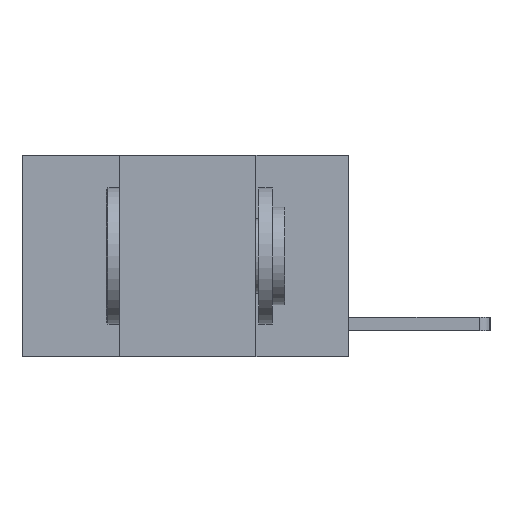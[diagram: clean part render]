
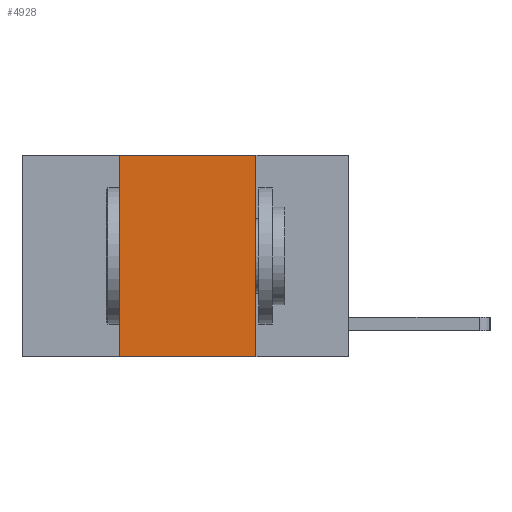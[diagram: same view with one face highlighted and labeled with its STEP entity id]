
A CAD part, left-side view. The second image highlights one B-rep face of the part: STEP entity #4928.
In plain terms, the highlighted planar face has unit normal (-1, 0, 0).
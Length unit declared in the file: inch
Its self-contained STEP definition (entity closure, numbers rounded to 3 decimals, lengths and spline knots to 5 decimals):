
#73 = LINE ( 'NONE', #692, #1565 ) ;
#147 = FACE_OUTER_BOUND ( 'NONE', #487, .T. ) ;
#232 = CARTESIAN_POINT ( 'NONE',  ( 0., 0.17, -0.37 ) ) ;
#289 = VECTOR ( 'NONE', #7069, 39.37008 ) ;
#487 = EDGE_LOOP ( 'NONE', ( #6045, #1967, #5439, #995 ) ) ;
#692 = CARTESIAN_POINT ( 'NONE',  ( 0., 0.6, -0.37 ) ) ;
#914 = CARTESIAN_POINT ( 'NONE',  ( 0., 0.42, 0. ) ) ;
#995 = ORIENTED_EDGE ( 'NONE', *, *, #9136, .T. ) ;
#1062 = CARTESIAN_POINT ( 'NONE',  ( 0., 0.42, -0.37 ) ) ;
#1565 = VECTOR ( 'NONE', #9286, 39.37008 ) ;
#1613 = DIRECTION ( 'NONE',  ( 0., -1., 0. ) ) ;
#1662 = VECTOR ( 'NONE', #1613, 39.37008 ) ;
#1663 = VERTEX_POINT ( 'NONE', #232 ) ;
#1890 = CARTESIAN_POINT ( 'NONE',  ( 0., 0.42, 0. ) ) ;
#1967 = ORIENTED_EDGE ( 'NONE', *, *, #4023, .F. ) ;
#2068 = CARTESIAN_POINT ( 'NONE',  ( 0., 0.6, 0. ) ) ;
#2085 = CARTESIAN_POINT ( 'NONE',  ( 0., 0.17, 0. ) ) ;
#2254 = LINE ( 'NONE', #2085, #289 ) ;
#2810 = DIRECTION ( 'NONE',  ( 0., 0., -1. ) ) ;
#3394 = VECTOR ( 'NONE', #7603, 39.37008 ) ;
#3487 = PLANE ( 'NONE',  #8303 ) ;
#3610 = LINE ( 'NONE', #1890, #3394 ) ;
#3615 = EDGE_CURVE ( 'NONE', #5662, #9301, #3610, .T. ) ;
#3793 = EDGE_CURVE ( 'NONE', #8738, #1663, #2254, .T. ) ;
#4023 = EDGE_CURVE ( 'NONE', #9301, #8738, #9252, .T. ) ;
#4590 = CARTESIAN_POINT ( 'NONE',  ( 0., 0.17, 0. ) ) ;
#4928 = ADVANCED_FACE ( 'NONE', ( #147 ), #3487, .F. ) ;
#5439 = ORIENTED_EDGE ( 'NONE', *, *, #3615, .F. ) ;
#5662 = VERTEX_POINT ( 'NONE', #1062 ) ;
#6045 = ORIENTED_EDGE ( 'NONE', *, *, #3793, .F. ) ;
#7052 = DIRECTION ( 'NONE',  ( 1., 0., 0. ) ) ;
#7069 = DIRECTION ( 'NONE',  ( 0., 0., -1. ) ) ;
#7603 = DIRECTION ( 'NONE',  ( 0., 0., 1. ) ) ;
#8303 = AXIS2_PLACEMENT_3D ( 'NONE', #2068, #7052, #2810 ) ;
#8738 = VERTEX_POINT ( 'NONE', #4590 ) ;
#8748 = CARTESIAN_POINT ( 'NONE',  ( 0., 0.6, 0. ) ) ;
#9136 = EDGE_CURVE ( 'NONE', #5662, #1663, #73, .T. ) ;
#9252 = LINE ( 'NONE', #8748, #1662 ) ;
#9286 = DIRECTION ( 'NONE',  ( 0., -1., 0. ) ) ;
#9301 = VERTEX_POINT ( 'NONE', #914 ) ;
